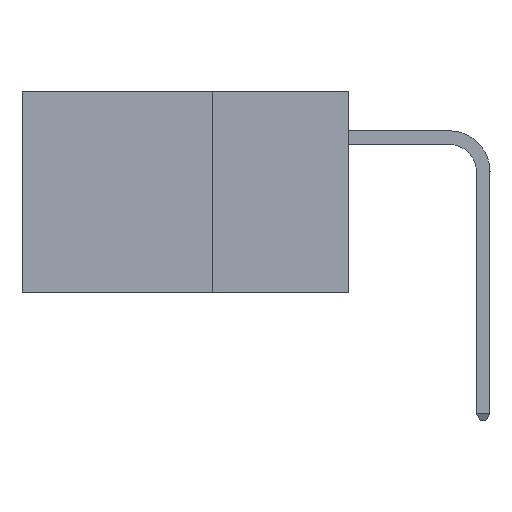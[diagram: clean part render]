
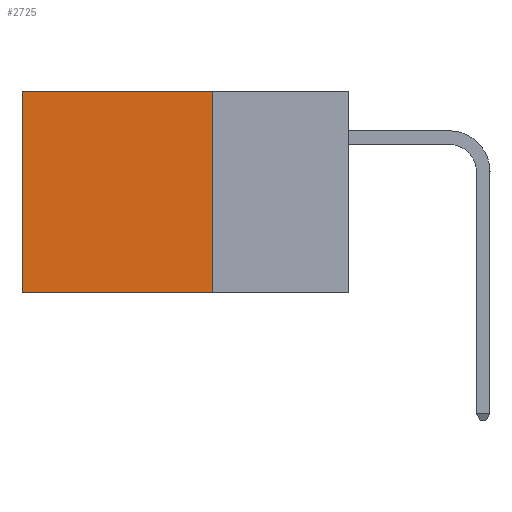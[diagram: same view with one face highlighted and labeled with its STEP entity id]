
A CAD part, left-side view. The second image highlights one B-rep face of the part: STEP entity #2725.
In plain terms, the highlighted planar face has unit normal (-1, 0, 0).
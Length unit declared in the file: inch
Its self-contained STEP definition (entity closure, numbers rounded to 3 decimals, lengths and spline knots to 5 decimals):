
#329 = ORIENTED_EDGE ( 'NONE', *, *, #21814, .F. ) ;
#2566 = ORIENTED_EDGE ( 'NONE', *, *, #34298, .T. ) ;
#2725 = ADVANCED_FACE ( 'NONE', ( #40339 ), #17381, .F. ) ;
#3976 = CARTESIAN_POINT ( 'NONE',  ( 0.2875, 0.6, 0. ) ) ;
#4248 = AXIS2_PLACEMENT_3D ( 'NONE', #34722, #41501, #37894 ) ;
#7338 = VECTOR ( 'NONE', #42034, 39.37008 ) ;
#9796 = VERTEX_POINT ( 'NONE', #30937 ) ;
#10007 = ORIENTED_EDGE ( 'NONE', *, *, #32064, .F. ) ;
#10724 = CARTESIAN_POINT ( 'NONE',  ( 0.2875, 0.25, 0. ) ) ;
#11063 = DIRECTION ( 'NONE',  ( 0., 0., -1. ) ) ;
#13109 = LINE ( 'NONE', #28917, #23333 ) ;
#14362 = CARTESIAN_POINT ( 'NONE',  ( 0.2875, 0.6, 0. ) ) ;
#17097 = DIRECTION ( 'NONE',  ( 0., 1., 0. ) ) ;
#17381 = PLANE ( 'NONE',  #4248 ) ;
#21485 = EDGE_LOOP ( 'NONE', ( #25378, #329, #10007, #2566 ) ) ;
#21814 = EDGE_CURVE ( 'NONE', #9796, #22318, #34233, .T. ) ;
#22137 = DIRECTION ( 'NONE',  ( 0., 1., 0. ) ) ;
#22318 = VERTEX_POINT ( 'NONE', #25827 ) ;
#22935 = VERTEX_POINT ( 'NONE', #26199 ) ;
#23333 = VECTOR ( 'NONE', #22137, 39.37008 ) ;
#24663 = VERTEX_POINT ( 'NONE', #14362 ) ;
#25378 = ORIENTED_EDGE ( 'NONE', *, *, #28929, .T. ) ;
#25827 = CARTESIAN_POINT ( 'NONE',  ( 0.2875, 0.6, -0.37 ) ) ;
#26199 = CARTESIAN_POINT ( 'NONE',  ( 0.2875, 0.25, 0. ) ) ;
#27260 = LINE ( 'NONE', #3976, #33183 ) ;
#28917 = CARTESIAN_POINT ( 'NONE',  ( 0.2875, 0.25, 0. ) ) ;
#28929 = EDGE_CURVE ( 'NONE', #24663, #22318, #27260, .T. ) ;
#30937 = CARTESIAN_POINT ( 'NONE',  ( 0.2875, 0.25, -0.37 ) ) ;
#32064 = EDGE_CURVE ( 'NONE', #22935, #9796, #32663, .T. ) ;
#32663 = LINE ( 'NONE', #10724, #7338 ) ;
#33183 = VECTOR ( 'NONE', #11063, 39.37008 ) ;
#33689 = CARTESIAN_POINT ( 'NONE',  ( 0.2875, 0.25, -0.37 ) ) ;
#34233 = LINE ( 'NONE', #33689, #34791 ) ;
#34298 = EDGE_CURVE ( 'NONE', #22935, #24663, #13109, .T. ) ;
#34722 = CARTESIAN_POINT ( 'NONE',  ( 0.2875, 0.25, 0. ) ) ;
#34791 = VECTOR ( 'NONE', #17097, 39.37008 ) ;
#37894 = DIRECTION ( 'NONE',  ( 0., 0., -1. ) ) ;
#40339 = FACE_OUTER_BOUND ( 'NONE', #21485, .T. ) ;
#41501 = DIRECTION ( 'NONE',  ( 1., 0., 0. ) ) ;
#42034 = DIRECTION ( 'NONE',  ( 0., 0., -1. ) ) ;
